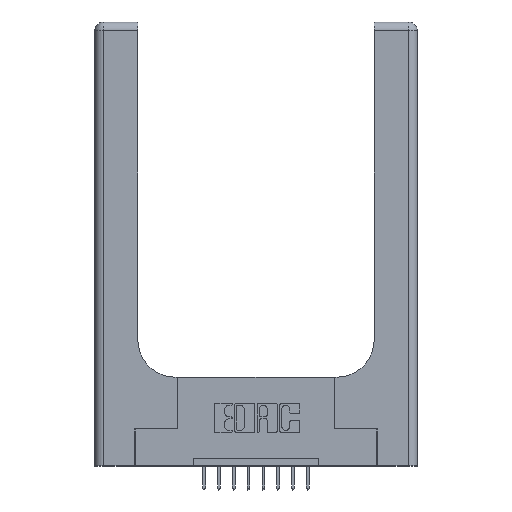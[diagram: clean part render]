
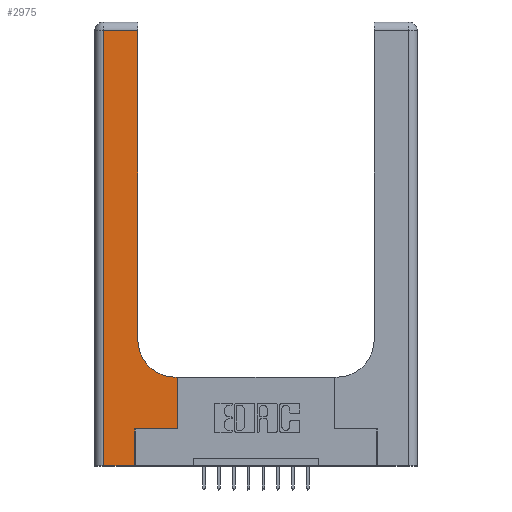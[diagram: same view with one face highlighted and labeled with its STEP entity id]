
A CAD part, top view. The second image highlights one B-rep face of the part: STEP entity #2975.
In plain terms, the highlighted planar face has unit normal (0, 0, 1).
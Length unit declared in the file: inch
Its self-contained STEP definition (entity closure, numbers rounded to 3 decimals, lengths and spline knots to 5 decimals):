
#192 = FACE_OUTER_BOUND ( 'NONE', #1332, .T. ) ;
#339 = ORIENTED_EDGE ( 'NONE', *, *, #2025, .T. ) ;
#453 = DIRECTION ( 'NONE',  ( 0., -1., 0. ) ) ;
#644 = EDGE_CURVE ( 'NONE', #15641, #4596, #820, .T. ) ;
#820 = LINE ( 'NONE', #14998, #7513 ) ;
#823 = VECTOR ( 'NONE', #10031, 39.37008 ) ;
#1076 = CARTESIAN_POINT ( 'NONE',  ( 0.5585, 0.25, 0.37 ) ) ;
#1141 = EDGE_CURVE ( 'NONE', #9455, #6419, #8110, .T. ) ;
#1263 = DIRECTION ( 'NONE',  ( 0., 0., -1. ) ) ;
#1332 = EDGE_LOOP ( 'NONE', ( #10761, #11677, #7758, #10468, #339, #9150, #12785, #15514, #10490 ) ) ;
#1524 = DIRECTION ( 'NONE',  ( 1., 0., 0. ) ) ;
#1613 = VERTEX_POINT ( 'NONE', #13914 ) ;
#1766 = CARTESIAN_POINT ( 'NONE',  ( 0.2915, 0.85, 0.37 ) ) ;
#2025 = EDGE_CURVE ( 'NONE', #4596, #5305, #3812, .T. ) ;
#2290 = CARTESIAN_POINT ( 'NONE',  ( 0.5415, 0.85, 0.37 ) ) ;
#2519 = CARTESIAN_POINT ( 'NONE',  ( 0.2915, 0.6, 0.37 ) ) ;
#2871 = CIRCLE ( 'NONE', #13420, 0.25 ) ;
#2975 = ADVANCED_FACE ( 'NONE', ( #192 ), #3434, .F. ) ;
#3021 = EDGE_CURVE ( 'NONE', #1613, #13424, #14334, .T. ) ;
#3233 = CARTESIAN_POINT ( 'NONE',  ( 0.269, 0.25, 0.37 ) ) ;
#3434 = PLANE ( 'NONE',  #5713 ) ;
#3812 = LINE ( 'NONE', #5807, #10154 ) ;
#3990 = CARTESIAN_POINT ( 'NONE',  ( 0.06, 2.94, 0.37 ) ) ;
#4280 = LINE ( 'NONE', #1076, #10793 ) ;
#4452 = VECTOR ( 'NONE', #453, 39.37008 ) ;
#4520 = VECTOR ( 'NONE', #6983, 39.37008 ) ;
#4596 = VERTEX_POINT ( 'NONE', #14401 ) ;
#4822 = CARTESIAN_POINT ( 'NONE',  ( 0.2915, 2.94, 0.37 ) ) ;
#5305 = VERTEX_POINT ( 'NONE', #3233 ) ;
#5552 = CARTESIAN_POINT ( 'NONE',  ( 0.5585, 0.25, 0.37 ) ) ;
#5713 = AXIS2_PLACEMENT_3D ( 'NONE', #14475, #6744, #7285 ) ;
#5807 = CARTESIAN_POINT ( 'NONE',  ( 0.269, 0., 0.37 ) ) ;
#6419 = VERTEX_POINT ( 'NONE', #3990 ) ;
#6744 = DIRECTION ( 'NONE',  ( 0., 0., -1. ) ) ;
#6833 = EDGE_CURVE ( 'NONE', #13424, #13464, #2871, .T. ) ;
#6983 = DIRECTION ( 'NONE',  ( 1., 0., 0. ) ) ;
#7285 = DIRECTION ( 'NONE',  ( -1., 0., 0. ) ) ;
#7513 = VECTOR ( 'NONE', #1524, 39.37008 ) ;
#7692 = DIRECTION ( 'NONE',  ( 0., 1., 0. ) ) ;
#7758 = ORIENTED_EDGE ( 'NONE', *, *, #11112, .T. ) ;
#7907 = EDGE_CURVE ( 'NONE', #13464, #9455, #13154, .T. ) ;
#8110 = LINE ( 'NONE', #13753, #823 ) ;
#8585 = DIRECTION ( 'NONE',  ( 1., 0., 0. ) ) ;
#9150 = ORIENTED_EDGE ( 'NONE', *, *, #14827, .T. ) ;
#9455 = VERTEX_POINT ( 'NONE', #4822 ) ;
#9611 = DIRECTION ( 'NONE',  ( 0., 1., 0. ) ) ;
#10020 = EDGE_CURVE ( 'NONE', #11825, #1613, #4280, .T. ) ;
#10031 = DIRECTION ( 'NONE',  ( -1., 0., 0. ) ) ;
#10154 = VECTOR ( 'NONE', #13143, 39.37008 ) ;
#10468 = ORIENTED_EDGE ( 'NONE', *, *, #644, .T. ) ;
#10490 = ORIENTED_EDGE ( 'NONE', *, *, #6833, .T. ) ;
#10719 = CARTESIAN_POINT ( 'NONE',  ( 0.5415, 0.6, 0.37 ) ) ;
#10761 = ORIENTED_EDGE ( 'NONE', *, *, #7907, .T. ) ;
#10793 = VECTOR ( 'NONE', #9611, 39.37008 ) ;
#11112 = EDGE_CURVE ( 'NONE', #6419, #15641, #12336, .T. ) ;
#11677 = ORIENTED_EDGE ( 'NONE', *, *, #1141, .T. ) ;
#11825 = VERTEX_POINT ( 'NONE', #5552 ) ;
#12181 = CARTESIAN_POINT ( 'NONE',  ( 0.2915, 3., 0.37 ) ) ;
#12236 = VECTOR ( 'NONE', #14740, 39.37008 ) ;
#12336 = LINE ( 'NONE', #15102, #4452 ) ;
#12785 = ORIENTED_EDGE ( 'NONE', *, *, #10020, .T. ) ;
#13143 = DIRECTION ( 'NONE',  ( 0., 1., 0. ) ) ;
#13154 = LINE ( 'NONE', #12181, #13926 ) ;
#13420 = AXIS2_PLACEMENT_3D ( 'NONE', #2290, #1263, #8585 ) ;
#13424 = VERTEX_POINT ( 'NONE', #10719 ) ;
#13464 = VERTEX_POINT ( 'NONE', #1766 ) ;
#13753 = CARTESIAN_POINT ( 'NONE',  ( 0., 2.94, 0.37 ) ) ;
#13914 = CARTESIAN_POINT ( 'NONE',  ( 0.5585, 0.6, 0.37 ) ) ;
#13926 = VECTOR ( 'NONE', #7692, 39.37008 ) ;
#14109 = LINE ( 'NONE', #14331, #4520 ) ;
#14331 = CARTESIAN_POINT ( 'NONE',  ( 0.269, 0.25, 0.37 ) ) ;
#14334 = LINE ( 'NONE', #2519, #12236 ) ;
#14401 = CARTESIAN_POINT ( 'NONE',  ( 0.269, 0., 0.37 ) ) ;
#14475 = CARTESIAN_POINT ( 'NONE',  ( 0., 3., 0.37 ) ) ;
#14666 = CARTESIAN_POINT ( 'NONE',  ( 0.06, 0., 0.37 ) ) ;
#14740 = DIRECTION ( 'NONE',  ( -1., 0., 0. ) ) ;
#14827 = EDGE_CURVE ( 'NONE', #5305, #11825, #14109, .T. ) ;
#14998 = CARTESIAN_POINT ( 'NONE',  ( 0., 0., 0.37 ) ) ;
#15102 = CARTESIAN_POINT ( 'NONE',  ( 0.06, 3., 0.37 ) ) ;
#15514 = ORIENTED_EDGE ( 'NONE', *, *, #3021, .T. ) ;
#15641 = VERTEX_POINT ( 'NONE', #14666 ) ;
